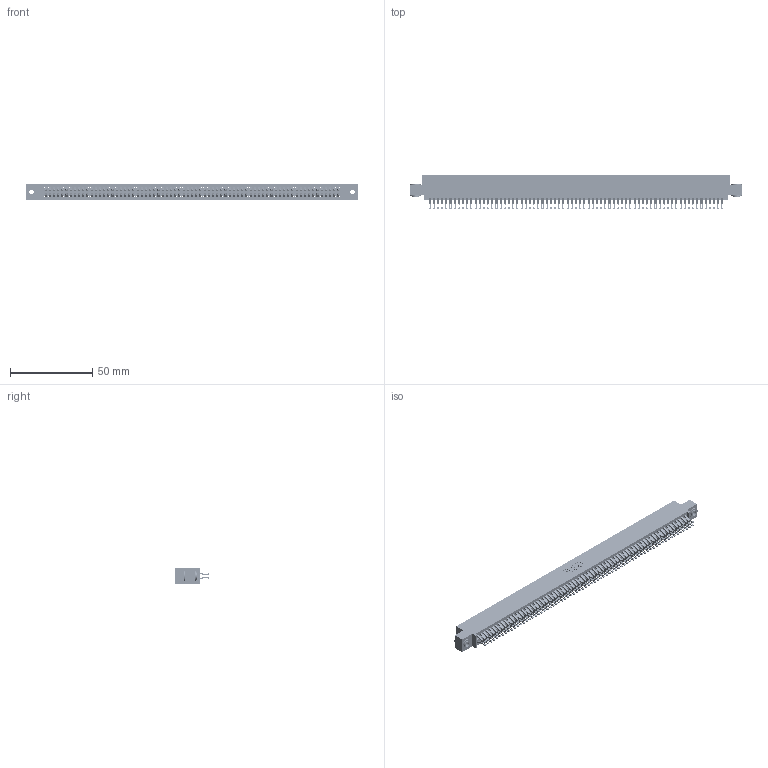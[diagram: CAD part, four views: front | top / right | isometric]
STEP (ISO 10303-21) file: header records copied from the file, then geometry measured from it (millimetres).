
FILE_DESCRIPTION (( 'STEP AP203' ), '1' );
FILE_NAME ('395-142-555-503.STEP', '2019-10-30T11:58:54', ( '' ), ( '' ), 'SwSTEP 2.0', 'SolidWorks 2016', '' );
FILE_SCHEMA (( 'CONFIG_CONTROL_DESIGN' ));
Length unit declared in the file: inch
Products named in the file (4): 345-292-001_555 Tail; 345-250-002_345-250-002-102; 395-142-555-503; 345 Part_0.110 Offset - 0.156 Dia-TH
Assembly tree (145 placements, depth 2):
  395-142-555-503
    345 Part_0.110 Offset - 0.156 Dia-TH
    345-292-001_555 Tail  x142
    345-250-002_345-250-002-102  x2
Bounding box: 201.55 x 21.13 x 9.4 mm (x, y, z)
Volume: 20205.8 mm3; surface area: 32159.5 mm2
Topology: 145 solids, 145 shells, 8120 faces, 25563 edges, 17038 vertices
Faces by surface type: plane 4496, cylinder 3616, cone 8
Entity records: 52912 total; most frequent: CARTESIAN_POINT 8853, ORIENTED_EDGE 8750, DIRECTION 7769, EDGE_CURVE 4375, LINE 3915, VECTOR 3915, VERTEX_POINT 2914, AXIS2_PLACEMENT_3D 1927
